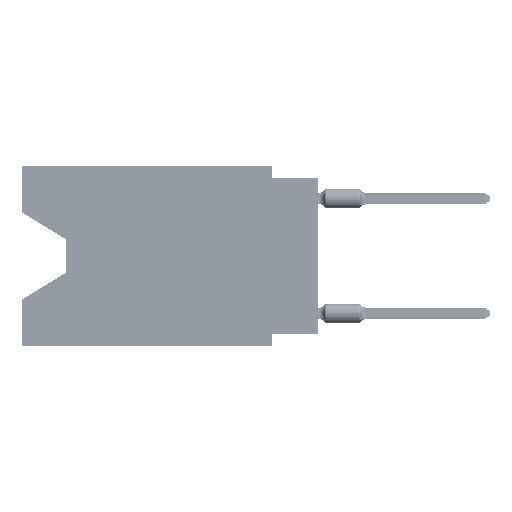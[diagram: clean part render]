
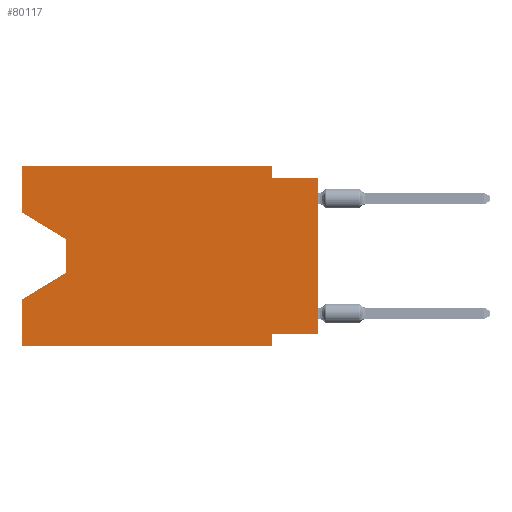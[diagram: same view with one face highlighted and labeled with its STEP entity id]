
A CAD part, left-side view. The second image highlights one B-rep face of the part: STEP entity #80117.
In plain terms, the highlighted planar face has unit normal (-1, 0, 0).
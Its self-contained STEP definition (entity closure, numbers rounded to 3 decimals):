
#132 = CARTESIAN_POINT ( 'NONE',  ( 0., 16.383, -9.906 ) ) ;
#757 = EDGE_CURVE ( 'NONE', #40082, #44026, #9555, .T. ) ;
#1624 = CARTESIAN_POINT ( 'NONE',  ( 0., 16.383, -2.546 ) ) ;
#2678 = ORIENTED_EDGE ( 'NONE', *, *, #5811, .F. ) ;
#3331 = DIRECTION ( 'NONE',  ( 0., 0.855, -0.519 ) ) ;
#3543 = CARTESIAN_POINT ( 'NONE',  ( 0., 16.383, 0. ) ) ;
#5811 = EDGE_CURVE ( 'NONE', #23034, #22115, #10564, .T. ) ;
#6181 = VERTEX_POINT ( 'NONE', #45868 ) ;
#7534 = CARTESIAN_POINT ( 'NONE',  ( 0., 0., -0.635 ) ) ;
#8639 = ORIENTED_EDGE ( 'NONE', *, *, #66989, .F. ) ;
#9381 = VERTEX_POINT ( 'NONE', #77528 ) ;
#9418 = LINE ( 'NONE', #41195, #71883 ) ;
#9555 = LINE ( 'NONE', #59942, #45603 ) ;
#9690 = DIRECTION ( 'NONE',  ( 0., 0., 1. ) ) ;
#10013 = DIRECTION ( 'NONE',  ( 0., 0., -1. ) ) ;
#10102 = LINE ( 'NONE', #48089, #81000 ) ;
#10564 = LINE ( 'NONE', #48149, #65691 ) ;
#10578 = VERTEX_POINT ( 'NONE', #78602 ) ;
#11156 = LINE ( 'NONE', #29747, #61121 ) ;
#11501 = EDGE_CURVE ( 'NONE', #6181, #42226, #9418, .T. ) ;
#16533 = DIRECTION ( 'NONE',  ( 0., 0., -1. ) ) ;
#16996 = ORIENTED_EDGE ( 'NONE', *, *, #58241, .F. ) ;
#18445 = ORIENTED_EDGE ( 'NONE', *, *, #11501, .F. ) ;
#20951 = CARTESIAN_POINT ( 'NONE',  ( 0., 2.54, -0.635 ) ) ;
#21059 = CARTESIAN_POINT ( 'NONE',  ( 0., 16.383, 0. ) ) ;
#21907 = CARTESIAN_POINT ( 'NONE',  ( 0., 13.97, -5.893 ) ) ;
#21992 = CARTESIAN_POINT ( 'NONE',  ( 0., 2.54, 0. ) ) ;
#22115 = VERTEX_POINT ( 'NONE', #41353 ) ;
#22196 = DIRECTION ( 'NONE',  ( 0., -1., 0. ) ) ;
#22660 = CARTESIAN_POINT ( 'NONE',  ( 0., 16.383, -7.36 ) ) ;
#22894 = EDGE_CURVE ( 'NONE', #42226, #61077, #78200, .T. ) ;
#23034 = VERTEX_POINT ( 'NONE', #61201 ) ;
#23338 = FACE_OUTER_BOUND ( 'NONE', #25224, .T. ) ;
#23879 = EDGE_CURVE ( 'NONE', #10578, #22115, #49335, .T. ) ;
#23889 = VECTOR ( 'NONE', #67724, 1000. ) ;
#24610 = DIRECTION ( 'NONE',  ( 0., 1., 0. ) ) ;
#25224 = EDGE_LOOP ( 'NONE', ( #73834, #50668, #32368, #28544, #48951, #2678, #8639, #61238, #55844, #38966, #18445, #16996 ) ) ;
#25412 = LINE ( 'NONE', #63020, #29585 ) ;
#28186 = EDGE_CURVE ( 'NONE', #61077, #42107, #48433, .T. ) ;
#28544 = ORIENTED_EDGE ( 'NONE', *, *, #34142, .F. ) ;
#29585 = VECTOR ( 'NONE', #24610, 1000. ) ;
#29747 = CARTESIAN_POINT ( 'NONE',  ( 0., 13.97, -4.013 ) ) ;
#32368 = ORIENTED_EDGE ( 'NONE', *, *, #757, .T. ) ;
#33854 = DIRECTION ( 'NONE',  ( 0., 0., 1. ) ) ;
#34142 = EDGE_CURVE ( 'NONE', #10578, #44026, #64997, .T. ) ;
#37636 = DIRECTION ( 'NONE',  ( 0., -1., 0. ) ) ;
#38966 = ORIENTED_EDGE ( 'NONE', *, *, #22894, .F. ) ;
#40082 = VERTEX_POINT ( 'NONE', #21907 ) ;
#41195 = CARTESIAN_POINT ( 'NONE',  ( 0., 16.383, 0. ) ) ;
#41353 = CARTESIAN_POINT ( 'NONE',  ( 0., 2.54, -9.906 ) ) ;
#42107 = VERTEX_POINT ( 'NONE', #7534 ) ;
#42226 = VERTEX_POINT ( 'NONE', #47572 ) ;
#42359 = DIRECTION ( 'NONE',  ( 1., 0., 0. ) ) ;
#42926 = CARTESIAN_POINT ( 'NONE',  ( 0., 16.383, 0. ) ) ;
#44026 = VERTEX_POINT ( 'NONE', #22660 ) ;
#44248 = VECTOR ( 'NONE', #58893, 1000. ) ;
#44422 = VECTOR ( 'NONE', #33854, 1000. ) ;
#45603 = VECTOR ( 'NONE', #3331, 1000. ) ;
#45868 = CARTESIAN_POINT ( 'NONE',  ( 0., 16.383, 0. ) ) ;
#46082 = EDGE_CURVE ( 'NONE', #72479, #9381, #51893, .T. ) ;
#47572 = CARTESIAN_POINT ( 'NONE',  ( 0., 2.54, 0. ) ) ;
#48089 = CARTESIAN_POINT ( 'NONE',  ( 0., 0., 0. ) ) ;
#48149 = CARTESIAN_POINT ( 'NONE',  ( 0., 2.54, -9.906 ) ) ;
#48433 = LINE ( 'NONE', #74841, #80182 ) ;
#48951 = ORIENTED_EDGE ( 'NONE', *, *, #23879, .T. ) ;
#49335 = LINE ( 'NONE', #132, #81086 ) ;
#50668 = ORIENTED_EDGE ( 'NONE', *, *, #78083, .T. ) ;
#51893 = LINE ( 'NONE', #65110, #44248 ) ;
#53240 = AXIS2_PLACEMENT_3D ( 'NONE', #3543, #42359, #54351 ) ;
#53437 = EDGE_CURVE ( 'NONE', #80115, #42107, #10102, .T. ) ;
#53553 = CARTESIAN_POINT ( 'NONE',  ( 0., 0., -9.271 ) ) ;
#54351 = DIRECTION ( 'NONE',  ( 0., 0., -1. ) ) ;
#55844 = ORIENTED_EDGE ( 'NONE', *, *, #28186, .F. ) ;
#58241 = EDGE_CURVE ( 'NONE', #72479, #6181, #77668, .T. ) ;
#58893 = DIRECTION ( 'NONE',  ( 0., -0.855, -0.519 ) ) ;
#59942 = CARTESIAN_POINT ( 'NONE',  ( 0., 13.97, -5.893 ) ) ;
#60540 = DIRECTION ( 'NONE',  ( 0., 0., -1. ) ) ;
#61077 = VERTEX_POINT ( 'NONE', #20951 ) ;
#61121 = VECTOR ( 'NONE', #16533, 1000. ) ;
#61201 = CARTESIAN_POINT ( 'NONE',  ( 0., 2.54, -9.271 ) ) ;
#61238 = ORIENTED_EDGE ( 'NONE', *, *, #53437, .T. ) ;
#63020 = CARTESIAN_POINT ( 'NONE',  ( 0., 0., -9.271 ) ) ;
#64997 = LINE ( 'NONE', #42926, #23889 ) ;
#65110 = CARTESIAN_POINT ( 'NONE',  ( 0., 16.383, -2.546 ) ) ;
#65691 = VECTOR ( 'NONE', #60540, 1000. ) ;
#66989 = EDGE_CURVE ( 'NONE', #80115, #23034, #25412, .T. ) ;
#67724 = DIRECTION ( 'NONE',  ( 0., 0., 1. ) ) ;
#71883 = VECTOR ( 'NONE', #22196, 1000. ) ;
#72479 = VERTEX_POINT ( 'NONE', #1624 ) ;
#73834 = ORIENTED_EDGE ( 'NONE', *, *, #46082, .T. ) ;
#74532 = DIRECTION ( 'NONE',  ( 0., -1., 0. ) ) ;
#74841 = CARTESIAN_POINT ( 'NONE',  ( 0., 0., -0.635 ) ) ;
#77528 = CARTESIAN_POINT ( 'NONE',  ( 0., 13.97, -4.013 ) ) ;
#77668 = LINE ( 'NONE', #21059, #44422 ) ;
#78083 = EDGE_CURVE ( 'NONE', #9381, #40082, #11156, .T. ) ;
#78200 = LINE ( 'NONE', #21992, #78341 ) ;
#78341 = VECTOR ( 'NONE', #10013, 1000. ) ;
#78602 = CARTESIAN_POINT ( 'NONE',  ( 0., 16.383, -9.906 ) ) ;
#79968 = PLANE ( 'NONE',  #53240 ) ;
#80115 = VERTEX_POINT ( 'NONE', #53553 ) ;
#80117 = ADVANCED_FACE ( 'NONE', ( #23338 ), #79968, .F. ) ;
#80182 = VECTOR ( 'NONE', #37636, 1000. ) ;
#81000 = VECTOR ( 'NONE', #9690, 1000. ) ;
#81086 = VECTOR ( 'NONE', #74532, 1000. ) ;
